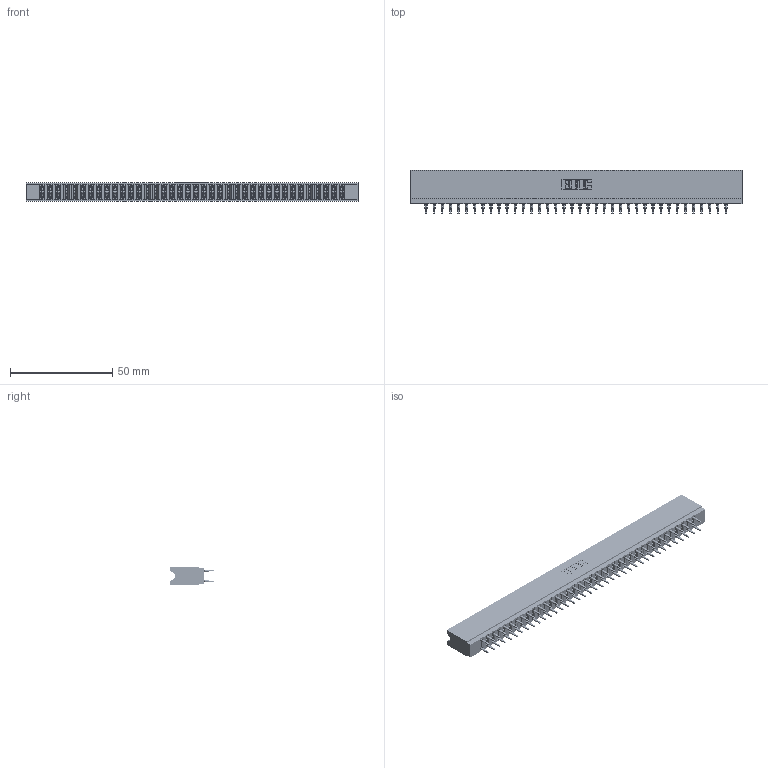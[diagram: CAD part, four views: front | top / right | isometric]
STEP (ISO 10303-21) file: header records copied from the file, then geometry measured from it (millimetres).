
FILE_DESCRIPTION (( 'STEP AP203' ), '1' );
FILE_NAME ('737-076-560-206.STEP', '2020-09-11T08:00:00', ( '' ), ( '' ), 'SwSTEP 2.0', 'SolidWorks 2020', '' );
FILE_SCHEMA (( 'CONFIG_CONTROL_DESIGN' ));
Length unit declared in the file: inch
Products named in the file (3): 745-292-001_560; 737-076-560-206; 737 Part_Insulator Option - 06
Assembly tree (77 placements, depth 2):
  737-076-560-206
    737 Part_Insulator Option - 06
    745-292-001_560  x76
Bounding box: 162.41 x 21.22 x 8.89 mm (x, y, z)
Volume: 16338.4 mm3; surface area: 25018.2 mm2
Topology: 77 solids, 77 shells, 7619 faces, 20853 edges, 13242 vertices
Faces by surface type: plane 3969, cylinder 1674, bspline 1520, torus 456
Entity records: 66090 total; most frequent: CARTESIAN_POINT 11978, ORIENTED_EDGE 11406, DIRECTION 9963, EDGE_CURVE 5703, LINE 5285, VECTOR 5285, VERTEX_POINT 3642, AXIS2_PLACEMENT_3D 2339
